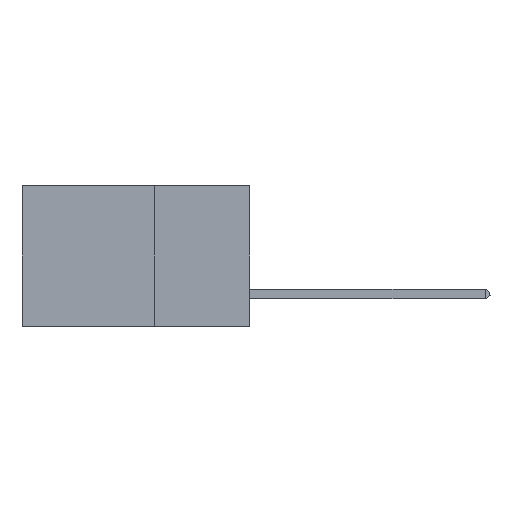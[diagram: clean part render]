
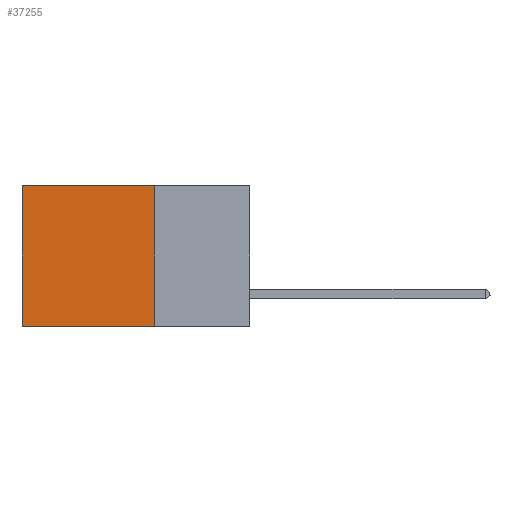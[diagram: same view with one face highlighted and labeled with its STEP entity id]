
A CAD part, left-side view. The second image highlights one B-rep face of the part: STEP entity #37255.
In plain terms, the highlighted planar face has unit normal (-1, 0, 0).
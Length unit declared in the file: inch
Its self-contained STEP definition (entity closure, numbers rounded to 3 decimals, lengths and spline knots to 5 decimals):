
#1358 = EDGE_LOOP ( 'NONE', ( #16351, #11026, #45333, #6803 ) ) ;
#1700 = LINE ( 'NONE', #11280, #12399 ) ;
#6803 = ORIENTED_EDGE ( 'NONE', *, *, #18370, .T. ) ;
#7283 = CARTESIAN_POINT ( 'NONE',  ( 0.2875, 0.25, 0. ) ) ;
#7497 = VECTOR ( 'NONE', #37488, 39.37008 ) ;
#9879 = EDGE_CURVE ( 'NONE', #41122, #34409, #34433, .T. ) ;
#11026 = ORIENTED_EDGE ( 'NONE', *, *, #20457, .F. ) ;
#11280 = CARTESIAN_POINT ( 'NONE',  ( 0.2875, 0.25, 0. ) ) ;
#12399 = VECTOR ( 'NONE', #18810, 39.37008 ) ;
#12746 = EDGE_CURVE ( 'NONE', #38740, #31940, #14938, .T. ) ;
#14938 = LINE ( 'NONE', #34977, #30547 ) ;
#16351 = ORIENTED_EDGE ( 'NONE', *, *, #9879, .T. ) ;
#18370 = EDGE_CURVE ( 'NONE', #38740, #41122, #1700, .T. ) ;
#18810 = DIRECTION ( 'NONE',  ( 0., 1., 0. ) ) ;
#20457 = EDGE_CURVE ( 'NONE', #31940, #34409, #44768, .T. ) ;
#22253 = CARTESIAN_POINT ( 'NONE',  ( 0.2875, 0.6, -0.37 ) ) ;
#26340 = DIRECTION ( 'NONE',  ( 0., 0., -1. ) ) ;
#30547 = VECTOR ( 'NONE', #46346, 39.37008 ) ;
#31940 = VERTEX_POINT ( 'NONE', #48082 ) ;
#33982 = FACE_OUTER_BOUND ( 'NONE', #1358, .T. ) ;
#34409 = VERTEX_POINT ( 'NONE', #22253 ) ;
#34433 = LINE ( 'NONE', #44668, #7497 ) ;
#34706 = DIRECTION ( 'NONE',  ( 1., 0., 0. ) ) ;
#34977 = CARTESIAN_POINT ( 'NONE',  ( 0.2875, 0.25, 0. ) ) ;
#37255 = ADVANCED_FACE ( 'NONE', ( #33982 ), #41739, .F. ) ;
#37488 = DIRECTION ( 'NONE',  ( 0., 0., -1. ) ) ;
#38740 = VERTEX_POINT ( 'NONE', #43592 ) ;
#41122 = VERTEX_POINT ( 'NONE', #42854 ) ;
#41739 = PLANE ( 'NONE',  #45263 ) ;
#42854 = CARTESIAN_POINT ( 'NONE',  ( 0.2875, 0.6, 0. ) ) ;
#43592 = CARTESIAN_POINT ( 'NONE',  ( 0.2875, 0.25, 0. ) ) ;
#44668 = CARTESIAN_POINT ( 'NONE',  ( 0.2875, 0.6, 0. ) ) ;
#44768 = LINE ( 'NONE', #46459, #49604 ) ;
#45263 = AXIS2_PLACEMENT_3D ( 'NONE', #7283, #34706, #26340 ) ;
#45333 = ORIENTED_EDGE ( 'NONE', *, *, #12746, .F. ) ;
#46346 = DIRECTION ( 'NONE',  ( 0., 0., -1. ) ) ;
#46459 = CARTESIAN_POINT ( 'NONE',  ( 0.2875, 0.25, -0.37 ) ) ;
#46790 = DIRECTION ( 'NONE',  ( 0., 1., 0. ) ) ;
#48082 = CARTESIAN_POINT ( 'NONE',  ( 0.2875, 0.25, -0.37 ) ) ;
#49604 = VECTOR ( 'NONE', #46790, 39.37008 ) ;
